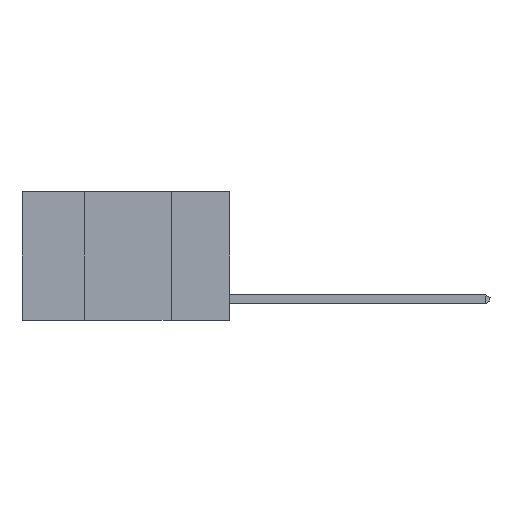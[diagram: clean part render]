
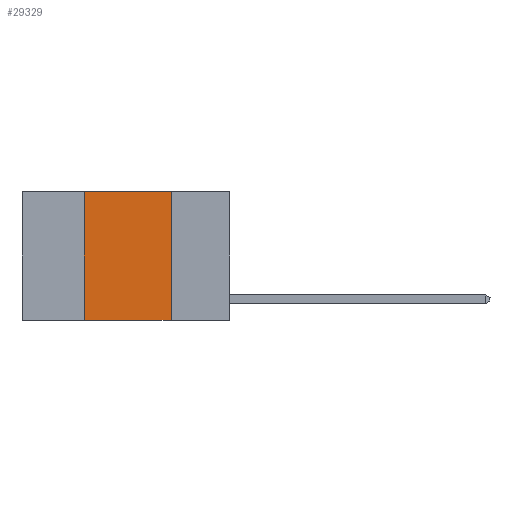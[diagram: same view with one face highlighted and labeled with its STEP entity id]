
A CAD part, left-side view. The second image highlights one B-rep face of the part: STEP entity #29329.
In plain terms, the highlighted planar face has unit normal (-1, 0, 0).
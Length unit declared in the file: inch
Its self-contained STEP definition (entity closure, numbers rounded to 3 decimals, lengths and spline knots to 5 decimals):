
#506 = FACE_OUTER_BOUND ( 'NONE', #16418, .T. ) ;
#1804 = DIRECTION ( 'NONE',  ( 0., 0., -1. ) ) ;
#2286 = ORIENTED_EDGE ( 'NONE', *, *, #20944, .T. ) ;
#2487 = CARTESIAN_POINT ( 'NONE',  ( 0., 0.6, -0.37 ) ) ;
#2928 = CARTESIAN_POINT ( 'NONE',  ( 0., 0.17, -0.37 ) ) ;
#3146 = EDGE_CURVE ( 'NONE', #26503, #26408, #8671, .T. ) ;
#3951 = VERTEX_POINT ( 'NONE', #22540 ) ;
#4720 = DIRECTION ( 'NONE',  ( 0., -1., 0. ) ) ;
#6919 = VECTOR ( 'NONE', #4720, 39.37008 ) ;
#7937 = ORIENTED_EDGE ( 'NONE', *, *, #23088, .F. ) ;
#8671 = LINE ( 'NONE', #15739, #9238 ) ;
#9140 = EDGE_CURVE ( 'NONE', #3951, #10643, #9971, .T. ) ;
#9238 = VECTOR ( 'NONE', #1804, 39.37008 ) ;
#9971 = LINE ( 'NONE', #20123, #14228 ) ;
#10643 = VERTEX_POINT ( 'NONE', #18523 ) ;
#13017 = CARTESIAN_POINT ( 'NONE',  ( 0., 0.6, 0. ) ) ;
#13402 = ORIENTED_EDGE ( 'NONE', *, *, #9140, .F. ) ;
#14228 = VECTOR ( 'NONE', #15511, 39.37008 ) ;
#15511 = DIRECTION ( 'NONE',  ( 0., 0., 1. ) ) ;
#15739 = CARTESIAN_POINT ( 'NONE',  ( 0., 0.17, 0. ) ) ;
#16418 = EDGE_LOOP ( 'NONE', ( #18722, #7937, #13402, #2286 ) ) ;
#16484 = VECTOR ( 'NONE', #19606, 39.37008 ) ;
#18523 = CARTESIAN_POINT ( 'NONE',  ( 0., 0.42, 0. ) ) ;
#18576 = AXIS2_PLACEMENT_3D ( 'NONE', #26094, #21302, #27868 ) ;
#18722 = ORIENTED_EDGE ( 'NONE', *, *, #3146, .F. ) ;
#19606 = DIRECTION ( 'NONE',  ( 0., -1., 0. ) ) ;
#20123 = CARTESIAN_POINT ( 'NONE',  ( 0., 0.42, 0. ) ) ;
#20944 = EDGE_CURVE ( 'NONE', #3951, #26408, #22829, .T. ) ;
#21302 = DIRECTION ( 'NONE',  ( 1., 0., 0. ) ) ;
#21630 = CARTESIAN_POINT ( 'NONE',  ( 0., 0.17, 0. ) ) ;
#22540 = CARTESIAN_POINT ( 'NONE',  ( 0., 0.42, -0.37 ) ) ;
#22829 = LINE ( 'NONE', #2487, #6919 ) ;
#23088 = EDGE_CURVE ( 'NONE', #10643, #26503, #26192, .T. ) ;
#25645 = PLANE ( 'NONE',  #18576 ) ;
#26094 = CARTESIAN_POINT ( 'NONE',  ( 0., 0.6, 0. ) ) ;
#26192 = LINE ( 'NONE', #13017, #16484 ) ;
#26408 = VERTEX_POINT ( 'NONE', #2928 ) ;
#26503 = VERTEX_POINT ( 'NONE', #21630 ) ;
#27868 = DIRECTION ( 'NONE',  ( 0., 0., -1. ) ) ;
#29329 = ADVANCED_FACE ( 'NONE', ( #506 ), #25645, .F. ) ;
